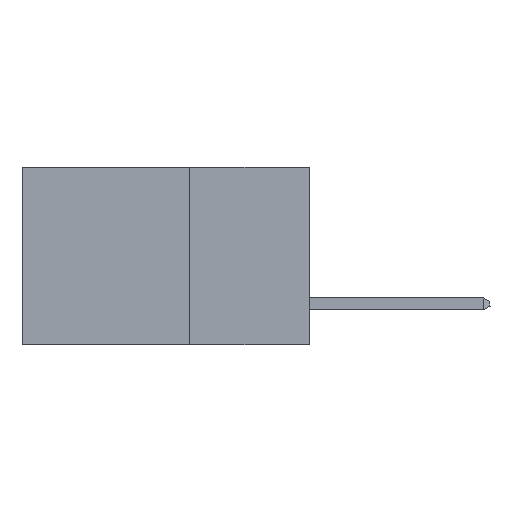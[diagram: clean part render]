
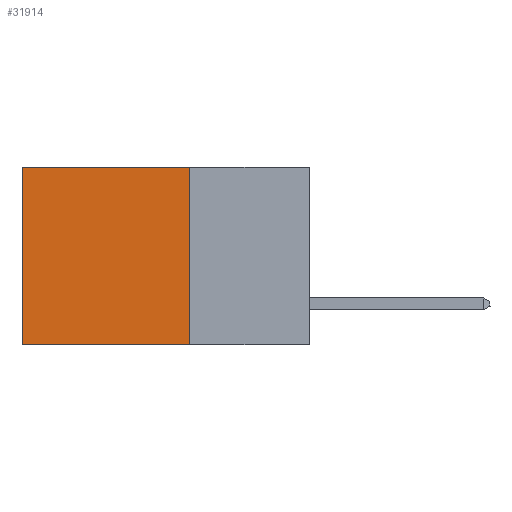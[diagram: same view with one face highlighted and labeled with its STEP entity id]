
A CAD part, left-side view. The second image highlights one B-rep face of the part: STEP entity #31914.
In plain terms, the highlighted planar face has unit normal (-1, 0, 0).
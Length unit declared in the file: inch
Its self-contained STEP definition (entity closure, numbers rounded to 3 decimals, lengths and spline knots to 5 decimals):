
#1373 = DIRECTION ( 'NONE',  ( 0., 1., 0. ) ) ;
#1390 = VERTEX_POINT ( 'NONE', #26421 ) ;
#2190 = CARTESIAN_POINT ( 'NONE',  ( 0.2875, 0.6, 0. ) ) ;
#2385 = CARTESIAN_POINT ( 'NONE',  ( 0.2875, 0.25, 0. ) ) ;
#2491 = LINE ( 'NONE', #2385, #3365 ) ;
#3365 = VECTOR ( 'NONE', #14283, 39.37008 ) ;
#3504 = CARTESIAN_POINT ( 'NONE',  ( 0.2875, 0.25, -0.37 ) ) ;
#4684 = CARTESIAN_POINT ( 'NONE',  ( 0.2875, 0.25, 0. ) ) ;
#5476 = CARTESIAN_POINT ( 'NONE',  ( 0.2875, 0.25, -0.37 ) ) ;
#5530 = ORIENTED_EDGE ( 'NONE', *, *, #28077, .F. ) ;
#7585 = CARTESIAN_POINT ( 'NONE',  ( 0.2875, 0.25, 0. ) ) ;
#7990 = PLANE ( 'NONE',  #37293 ) ;
#9064 = VECTOR ( 'NONE', #10849, 39.37008 ) ;
#9452 = DIRECTION ( 'NONE',  ( 0., 1., 0. ) ) ;
#10849 = DIRECTION ( 'NONE',  ( 0., 0., -1. ) ) ;
#12451 = LINE ( 'NONE', #4684, #35240 ) ;
#14283 = DIRECTION ( 'NONE',  ( 0., 0., -1. ) ) ;
#14566 = ORIENTED_EDGE ( 'NONE', *, *, #18511, .T. ) ;
#16650 = LINE ( 'NONE', #3504, #20774 ) ;
#16767 = DIRECTION ( 'NONE',  ( 1., 0., 0. ) ) ;
#18511 = EDGE_CURVE ( 'NONE', #1390, #20019, #12451, .T. ) ;
#19563 = ORIENTED_EDGE ( 'NONE', *, *, #34113, .F. ) ;
#20019 = VERTEX_POINT ( 'NONE', #24747 ) ;
#20774 = VECTOR ( 'NONE', #9452, 39.37008 ) ;
#23379 = ORIENTED_EDGE ( 'NONE', *, *, #35818, .T. ) ;
#24747 = CARTESIAN_POINT ( 'NONE',  ( 0.2875, 0.6, 0. ) ) ;
#25172 = DIRECTION ( 'NONE',  ( 0., 0., -1. ) ) ;
#26376 = VERTEX_POINT ( 'NONE', #5476 ) ;
#26421 = CARTESIAN_POINT ( 'NONE',  ( 0.2875, 0.25, 0. ) ) ;
#28077 = EDGE_CURVE ( 'NONE', #1390, #26376, #2491, .T. ) ;
#28693 = EDGE_LOOP ( 'NONE', ( #23379, #19563, #5530, #14566 ) ) ;
#28909 = FACE_OUTER_BOUND ( 'NONE', #28693, .T. ) ;
#30304 = LINE ( 'NONE', #2190, #9064 ) ;
#31914 = ADVANCED_FACE ( 'NONE', ( #28909 ), #7990, .F. ) ;
#34113 = EDGE_CURVE ( 'NONE', #26376, #35130, #16650, .T. ) ;
#34596 = CARTESIAN_POINT ( 'NONE',  ( 0.2875, 0.6, -0.37 ) ) ;
#35130 = VERTEX_POINT ( 'NONE', #34596 ) ;
#35240 = VECTOR ( 'NONE', #1373, 39.37008 ) ;
#35818 = EDGE_CURVE ( 'NONE', #20019, #35130, #30304, .T. ) ;
#37293 = AXIS2_PLACEMENT_3D ( 'NONE', #7585, #16767, #25172 ) ;
